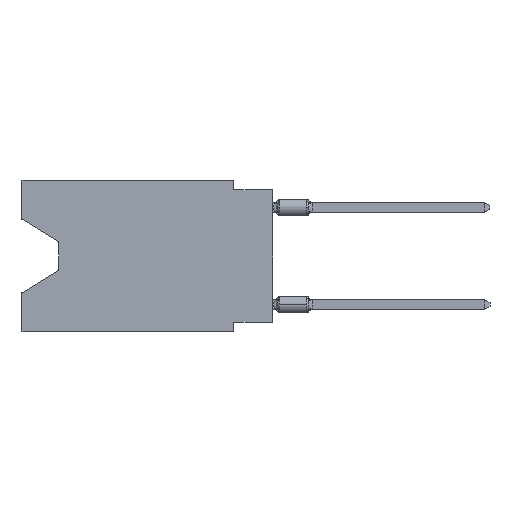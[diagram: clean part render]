
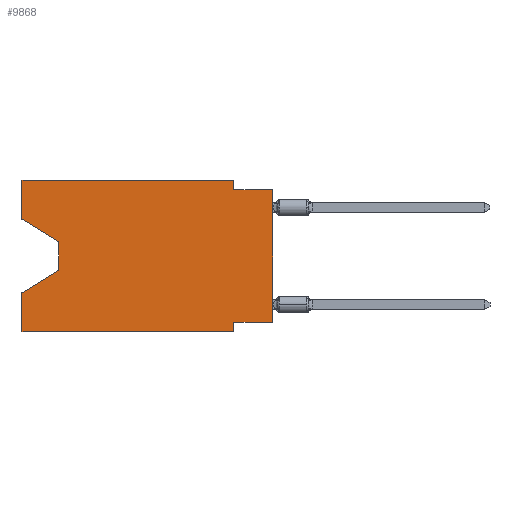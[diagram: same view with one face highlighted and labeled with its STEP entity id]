
A CAD part, left-side view. The second image highlights one B-rep face of the part: STEP entity #9868.
In plain terms, the highlighted planar face has unit normal (-1, 0, 0).
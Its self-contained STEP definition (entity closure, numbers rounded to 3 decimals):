
#478 = CARTESIAN_POINT ( 'NONE',  ( 0., 16.383, -2.546 ) ) ;
#488 = VECTOR ( 'NONE', #13449, 1000. ) ;
#691 = ORIENTED_EDGE ( 'NONE', *, *, #2967, .F. ) ;
#1139 = LINE ( 'NONE', #6126, #19229 ) ;
#1536 = EDGE_CURVE ( 'NONE', #10337, #8668, #7710, .T. ) ;
#1660 = VERTEX_POINT ( 'NONE', #11001 ) ;
#2853 = VECTOR ( 'NONE', #11235, 1000. ) ;
#2967 = EDGE_CURVE ( 'NONE', #12858, #22265, #5638, .T. ) ;
#3579 = DIRECTION ( 'NONE',  ( 1., 0., 0. ) ) ;
#4011 = VECTOR ( 'NONE', #14622, 1000. ) ;
#4127 = LINE ( 'NONE', #11033, #4011 ) ;
#4145 = ORIENTED_EDGE ( 'NONE', *, *, #6473, .F. ) ;
#4209 = LINE ( 'NONE', #7452, #2853 ) ;
#4215 = EDGE_CURVE ( 'NONE', #8880, #10337, #4479, .T. ) ;
#4255 = ORIENTED_EDGE ( 'NONE', *, *, #20844, .F. ) ;
#4479 = LINE ( 'NONE', #16233, #10345 ) ;
#4497 = DIRECTION ( 'NONE',  ( 0., -1., 0. ) ) ;
#4805 = CARTESIAN_POINT ( 'NONE',  ( 0., 2.54, -9.906 ) ) ;
#4929 = EDGE_CURVE ( 'NONE', #6749, #6605, #8711, .T. ) ;
#5382 = CARTESIAN_POINT ( 'NONE',  ( 0., 16.383, 0. ) ) ;
#5480 = AXIS2_PLACEMENT_3D ( 'NONE', #21327, #3579, #9233 ) ;
#5638 = LINE ( 'NONE', #6103, #15974 ) ;
#5871 = LINE ( 'NONE', #11278, #22754 ) ;
#5909 = LINE ( 'NONE', #478, #21384 ) ;
#6099 = CARTESIAN_POINT ( 'NONE',  ( 0., 13.97, -5.893 ) ) ;
#6103 = CARTESIAN_POINT ( 'NONE',  ( 0., 16.383, 0. ) ) ;
#6126 = CARTESIAN_POINT ( 'NONE',  ( 0., 16.383, 0. ) ) ;
#6133 = ORIENTED_EDGE ( 'NONE', *, *, #19735, .F. ) ;
#6177 = CARTESIAN_POINT ( 'NONE',  ( 0., 16.383, -2.546 ) ) ;
#6473 = EDGE_CURVE ( 'NONE', #1660, #8668, #4209, .T. ) ;
#6605 = VERTEX_POINT ( 'NONE', #9054 ) ;
#6618 = ORIENTED_EDGE ( 'NONE', *, *, #8644, .T. ) ;
#6743 = VECTOR ( 'NONE', #20028, 1000. ) ;
#6749 = VERTEX_POINT ( 'NONE', #7801 ) ;
#7067 = EDGE_CURVE ( 'NONE', #20332, #11295, #5871, .T. ) ;
#7452 = CARTESIAN_POINT ( 'NONE',  ( 0., 16.383, 0. ) ) ;
#7710 = LINE ( 'NONE', #6099, #6743 ) ;
#7734 = VERTEX_POINT ( 'NONE', #21096 ) ;
#7801 = CARTESIAN_POINT ( 'NONE',  ( 0., 0., -9.271 ) ) ;
#8023 = DIRECTION ( 'NONE',  ( 0., 0., -1. ) ) ;
#8478 = ORIENTED_EDGE ( 'NONE', *, *, #10338, .F. ) ;
#8621 = LINE ( 'NONE', #16913, #488 ) ;
#8644 = EDGE_CURVE ( 'NONE', #1660, #11295, #14017, .T. ) ;
#8668 = VERTEX_POINT ( 'NONE', #17373 ) ;
#8705 = VECTOR ( 'NONE', #8023, 1000. ) ;
#8711 = LINE ( 'NONE', #18105, #9971 ) ;
#8880 = VERTEX_POINT ( 'NONE', #12976 ) ;
#9054 = CARTESIAN_POINT ( 'NONE',  ( 0., 0., -0.635 ) ) ;
#9233 = DIRECTION ( 'NONE',  ( 0., 0., -1. ) ) ;
#9574 = ORIENTED_EDGE ( 'NONE', *, *, #4215, .T. ) ;
#9656 = CARTESIAN_POINT ( 'NONE',  ( 0., 13.97, -5.893 ) ) ;
#9868 = ADVANCED_FACE ( 'NONE', ( #15804 ), #14179, .F. ) ;
#9971 = VECTOR ( 'NONE', #20908, 1000. ) ;
#10337 = VERTEX_POINT ( 'NONE', #9656 ) ;
#10338 = EDGE_CURVE ( 'NONE', #6749, #20332, #4127, .T. ) ;
#10345 = VECTOR ( 'NONE', #12997, 1000. ) ;
#10729 = DIRECTION ( 'NONE',  ( 0., -0.855, -0.519 ) ) ;
#11001 = CARTESIAN_POINT ( 'NONE',  ( 0., 16.383, -9.906 ) ) ;
#11033 = CARTESIAN_POINT ( 'NONE',  ( 0., 0., -9.271 ) ) ;
#11235 = DIRECTION ( 'NONE',  ( 0., 0., 1. ) ) ;
#11278 = CARTESIAN_POINT ( 'NONE',  ( 0., 2.54, -9.906 ) ) ;
#11295 = VERTEX_POINT ( 'NONE', #4805 ) ;
#11664 = VECTOR ( 'NONE', #12182, 1000. ) ;
#12182 = DIRECTION ( 'NONE',  ( 0., -1., 0. ) ) ;
#12470 = ORIENTED_EDGE ( 'NONE', *, *, #1536, .T. ) ;
#12858 = VERTEX_POINT ( 'NONE', #6177 ) ;
#12883 = EDGE_CURVE ( 'NONE', #18896, #7734, #18503, .T. ) ;
#12976 = CARTESIAN_POINT ( 'NONE',  ( 0., 13.97, -4.013 ) ) ;
#12997 = DIRECTION ( 'NONE',  ( 0., 0., -1. ) ) ;
#13228 = DIRECTION ( 'NONE',  ( 0., 0., -1. ) ) ;
#13449 = DIRECTION ( 'NONE',  ( 0., -1., 0. ) ) ;
#13593 = EDGE_LOOP ( 'NONE', ( #19810, #9574, #12470, #4145, #6618, #14909, #8478, #19363, #4255, #17284, #6133, #691 ) ) ;
#13687 = CARTESIAN_POINT ( 'NONE',  ( 0., 16.383, -9.906 ) ) ;
#14017 = LINE ( 'NONE', #13687, #11664 ) ;
#14179 = PLANE ( 'NONE',  #5480 ) ;
#14622 = DIRECTION ( 'NONE',  ( 0., 1., 0. ) ) ;
#14909 = ORIENTED_EDGE ( 'NONE', *, *, #7067, .F. ) ;
#15716 = CARTESIAN_POINT ( 'NONE',  ( 0., 2.54, -9.271 ) ) ;
#15804 = FACE_OUTER_BOUND ( 'NONE', #13593, .T. ) ;
#15974 = VECTOR ( 'NONE', #16341, 1000. ) ;
#16233 = CARTESIAN_POINT ( 'NONE',  ( 0., 13.97, -4.013 ) ) ;
#16341 = DIRECTION ( 'NONE',  ( 0., 0., 1. ) ) ;
#16778 = CARTESIAN_POINT ( 'NONE',  ( 0., 2.54, 0. ) ) ;
#16913 = CARTESIAN_POINT ( 'NONE',  ( 0., 0., -0.635 ) ) ;
#17284 = ORIENTED_EDGE ( 'NONE', *, *, #12883, .F. ) ;
#17373 = CARTESIAN_POINT ( 'NONE',  ( 0., 16.383, -7.36 ) ) ;
#18023 = EDGE_CURVE ( 'NONE', #12858, #8880, #5909, .T. ) ;
#18105 = CARTESIAN_POINT ( 'NONE',  ( 0., 0., 0. ) ) ;
#18503 = LINE ( 'NONE', #16778, #8705 ) ;
#18896 = VERTEX_POINT ( 'NONE', #20447 ) ;
#19229 = VECTOR ( 'NONE', #4497, 1000. ) ;
#19363 = ORIENTED_EDGE ( 'NONE', *, *, #4929, .T. ) ;
#19735 = EDGE_CURVE ( 'NONE', #22265, #18896, #1139, .T. ) ;
#19810 = ORIENTED_EDGE ( 'NONE', *, *, #18023, .T. ) ;
#20028 = DIRECTION ( 'NONE',  ( 0., 0.855, -0.519 ) ) ;
#20332 = VERTEX_POINT ( 'NONE', #15716 ) ;
#20447 = CARTESIAN_POINT ( 'NONE',  ( 0., 2.54, 0. ) ) ;
#20844 = EDGE_CURVE ( 'NONE', #7734, #6605, #8621, .T. ) ;
#20908 = DIRECTION ( 'NONE',  ( 0., 0., 1. ) ) ;
#21096 = CARTESIAN_POINT ( 'NONE',  ( 0., 2.54, -0.635 ) ) ;
#21327 = CARTESIAN_POINT ( 'NONE',  ( 0., 16.383, 0. ) ) ;
#21384 = VECTOR ( 'NONE', #10729, 1000. ) ;
#22265 = VERTEX_POINT ( 'NONE', #5382 ) ;
#22754 = VECTOR ( 'NONE', #13228, 1000. ) ;
